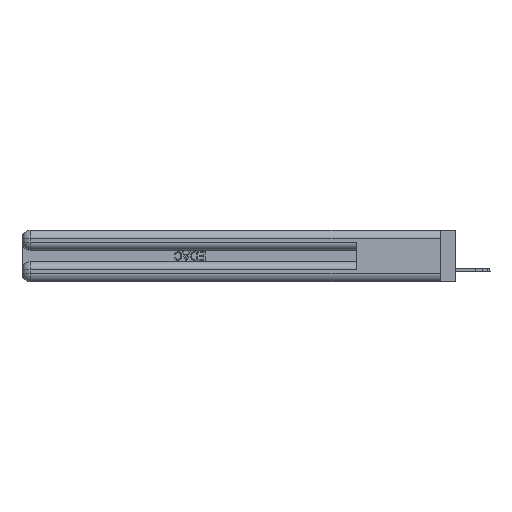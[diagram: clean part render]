
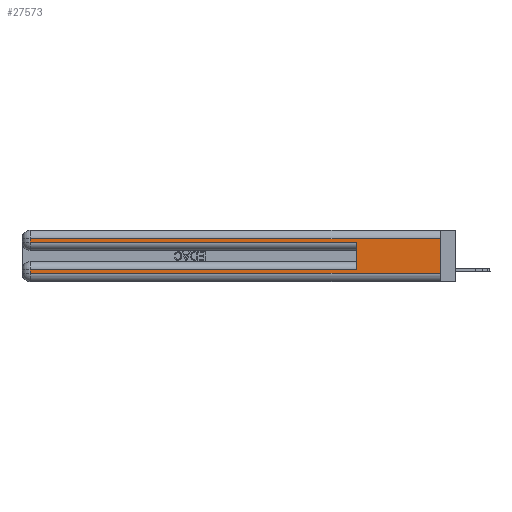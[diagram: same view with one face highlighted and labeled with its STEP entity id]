
A CAD part, left-side view. The second image highlights one B-rep face of the part: STEP entity #27573.
In plain terms, the highlighted planar face has unit normal (-1, 0, 0).
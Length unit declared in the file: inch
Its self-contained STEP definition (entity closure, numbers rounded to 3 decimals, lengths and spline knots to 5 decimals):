
#84 = CARTESIAN_POINT ( 'NONE',  ( 0., 0.6, 0.285 ) ) ;
#285 = LINE ( 'NONE', #27814, #13431 ) ;
#995 = EDGE_CURVE ( 'NONE', #12671, #9795, #18872, .T. ) ;
#1482 = DIRECTION ( 'NONE',  ( 1., 0., 0. ) ) ;
#1653 = DIRECTION ( 'NONE',  ( 0., -1., 0. ) ) ;
#1835 = CARTESIAN_POINT ( 'NONE',  ( 0., 2.94, 0.085 ) ) ;
#1878 = EDGE_CURVE ( 'NONE', #15830, #22567, #30682, .T. ) ;
#2512 = VERTEX_POINT ( 'NONE', #14715 ) ;
#2831 = LINE ( 'NONE', #27173, #5493 ) ;
#2914 = ORIENTED_EDGE ( 'NONE', *, *, #29937, .T. ) ;
#3276 = CARTESIAN_POINT ( 'NONE',  ( 0., 0., 0.31 ) ) ;
#5198 = ORIENTED_EDGE ( 'NONE', *, *, #28341, .T. ) ;
#5493 = VECTOR ( 'NONE', #1653, 39.37008 ) ;
#6583 = VECTOR ( 'NONE', #8356, 39.37008 ) ;
#7230 = PLANE ( 'NONE',  #21823 ) ;
#8356 = DIRECTION ( 'NONE',  ( 0., -1., 0. ) ) ;
#8385 = VERTEX_POINT ( 'NONE', #1835 ) ;
#9617 = DIRECTION ( 'NONE',  ( 0., 0., -1. ) ) ;
#9795 = VERTEX_POINT ( 'NONE', #35892 ) ;
#10047 = VERTEX_POINT ( 'NONE', #13498 ) ;
#11963 = VECTOR ( 'NONE', #16376, 39.37008 ) ;
#12358 = DIRECTION ( 'NONE',  ( 0., 0., -1. ) ) ;
#12671 = VERTEX_POINT ( 'NONE', #23853 ) ;
#13023 = ORIENTED_EDGE ( 'NONE', *, *, #34131, .F. ) ;
#13372 = EDGE_CURVE ( 'NONE', #8385, #13410, #29029, .T. ) ;
#13410 = VERTEX_POINT ( 'NONE', #18136 ) ;
#13431 = VECTOR ( 'NONE', #16462, 39.37008 ) ;
#13477 = VECTOR ( 'NONE', #25909, 39.37008 ) ;
#13498 = CARTESIAN_POINT ( 'NONE',  ( 0., 0.6, 0.085 ) ) ;
#13699 = ORIENTED_EDGE ( 'NONE', *, *, #14675, .T. ) ;
#14675 = EDGE_CURVE ( 'NONE', #12671, #2512, #19074, .T. ) ;
#14715 = CARTESIAN_POINT ( 'NONE',  ( 0., 2.94, 0.31 ) ) ;
#15409 = ORIENTED_EDGE ( 'NONE', *, *, #1878, .T. ) ;
#15613 = VECTOR ( 'NONE', #20434, 39.37008 ) ;
#15672 = ORIENTED_EDGE ( 'NONE', *, *, #995, .F. ) ;
#15830 = VERTEX_POINT ( 'NONE', #34491 ) ;
#16376 = DIRECTION ( 'NONE',  ( 0., 1., 0. ) ) ;
#16462 = DIRECTION ( 'NONE',  ( 0., 0., 1. ) ) ;
#16941 = LINE ( 'NONE', #31700, #13477 ) ;
#18136 = CARTESIAN_POINT ( 'NONE',  ( 0., 2.94, 0.06 ) ) ;
#18872 = LINE ( 'NONE', #28111, #33354 ) ;
#19074 = LINE ( 'NONE', #3276, #15613 ) ;
#19195 = CARTESIAN_POINT ( 'NONE',  ( 0., 0., 0.085 ) ) ;
#20434 = DIRECTION ( 'NONE',  ( 0., 1., 0. ) ) ;
#21636 = VECTOR ( 'NONE', #9617, 39.37008 ) ;
#21823 = AXIS2_PLACEMENT_3D ( 'NONE', #29815, #1482, #29461 ) ;
#21826 = CARTESIAN_POINT ( 'NONE',  ( 0., 0., 0.285 ) ) ;
#22288 = FACE_OUTER_BOUND ( 'NONE', #28483, .T. ) ;
#22567 = VERTEX_POINT ( 'NONE', #84 ) ;
#23853 = CARTESIAN_POINT ( 'NONE',  ( 0., 0., 0.31 ) ) ;
#24731 = LINE ( 'NONE', #19195, #11963 ) ;
#25909 = DIRECTION ( 'NONE',  ( 0., 0., -1. ) ) ;
#26325 = CARTESIAN_POINT ( 'NONE',  ( 0., 2.94, 0.37 ) ) ;
#26774 = ORIENTED_EDGE ( 'NONE', *, *, #30531, .T. ) ;
#27173 = CARTESIAN_POINT ( 'NONE',  ( 0., 0., 0.06 ) ) ;
#27573 = ADVANCED_FACE ( 'NONE', ( #22288 ), #7230, .F. ) ;
#27814 = CARTESIAN_POINT ( 'NONE',  ( 0., 0.6, 0.145 ) ) ;
#28111 = CARTESIAN_POINT ( 'NONE',  ( 0., 0., 0.37 ) ) ;
#28341 = EDGE_CURVE ( 'NONE', #2512, #15830, #16941, .T. ) ;
#28483 = EDGE_LOOP ( 'NONE', ( #15672, #13699, #5198, #15409, #13023, #26774, #31777, #2914 ) ) ;
#29029 = LINE ( 'NONE', #26325, #21636 ) ;
#29461 = DIRECTION ( 'NONE',  ( 0., 0., -1. ) ) ;
#29815 = CARTESIAN_POINT ( 'NONE',  ( 0., 0., 0.37 ) ) ;
#29937 = EDGE_CURVE ( 'NONE', #13410, #9795, #2831, .T. ) ;
#30531 = EDGE_CURVE ( 'NONE', #10047, #8385, #24731, .T. ) ;
#30682 = LINE ( 'NONE', #21826, #6583 ) ;
#31700 = CARTESIAN_POINT ( 'NONE',  ( 0., 2.94, 0.37 ) ) ;
#31777 = ORIENTED_EDGE ( 'NONE', *, *, #13372, .T. ) ;
#33354 = VECTOR ( 'NONE', #12358, 39.37008 ) ;
#34131 = EDGE_CURVE ( 'NONE', #10047, #22567, #285, .T. ) ;
#34491 = CARTESIAN_POINT ( 'NONE',  ( 0., 2.94, 0.285 ) ) ;
#35892 = CARTESIAN_POINT ( 'NONE',  ( 0., 0., 0.06 ) ) ;
